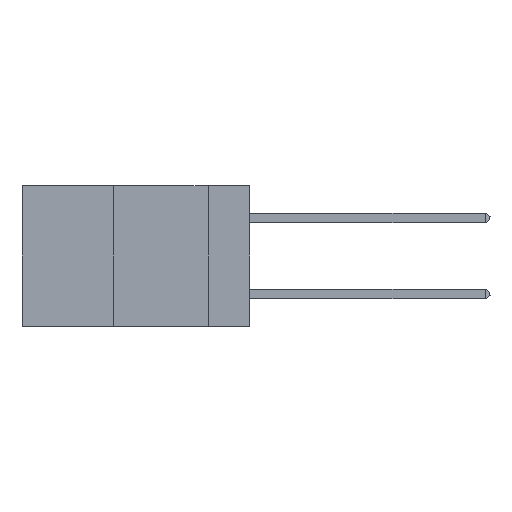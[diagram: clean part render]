
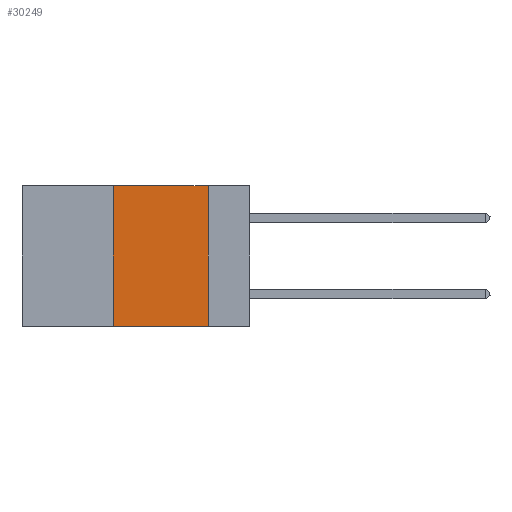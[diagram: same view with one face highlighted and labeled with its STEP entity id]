
A CAD part, left-side view. The second image highlights one B-rep face of the part: STEP entity #30249.
In plain terms, the highlighted planar face has unit normal (-1, 0, 0).
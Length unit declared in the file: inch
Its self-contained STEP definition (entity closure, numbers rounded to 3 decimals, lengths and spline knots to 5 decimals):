
#852 = VERTEX_POINT ( 'NONE', #10774 ) ;
#1862 = VERTEX_POINT ( 'NONE', #9289 ) ;
#2114 = CARTESIAN_POINT ( 'NONE',  ( 0., 0.11, -0.37 ) ) ;
#4923 = VECTOR ( 'NONE', #18340, 39.37008 ) ;
#6065 = CARTESIAN_POINT ( 'NONE',  ( 0., 0.11, 0. ) ) ;
#6107 = VERTEX_POINT ( 'NONE', #2114 ) ;
#6828 = VERTEX_POINT ( 'NONE', #16923 ) ;
#9289 = CARTESIAN_POINT ( 'NONE',  ( 0., 0.36, 0. ) ) ;
#10050 = ORIENTED_EDGE ( 'NONE', *, *, #13258, .F. ) ;
#10533 = LINE ( 'NONE', #11750, #4923 ) ;
#10774 = CARTESIAN_POINT ( 'NONE',  ( 0., 0.36, -0.37 ) ) ;
#11750 = CARTESIAN_POINT ( 'NONE',  ( 0., 0.6, 0. ) ) ;
#12560 = CARTESIAN_POINT ( 'NONE',  ( 0., 0.6, -0.37 ) ) ;
#13113 = CARTESIAN_POINT ( 'NONE',  ( 0., 0.6, 0. ) ) ;
#13258 = EDGE_CURVE ( 'NONE', #1862, #6828, #10533, .T. ) ;
#14888 = EDGE_CURVE ( 'NONE', #852, #6107, #37290, .T. ) ;
#16923 = CARTESIAN_POINT ( 'NONE',  ( 0., 0.11, 0. ) ) ;
#18340 = DIRECTION ( 'NONE',  ( 0., -1., 0. ) ) ;
#20455 = DIRECTION ( 'NONE',  ( 0., 0., -1. ) ) ;
#30249 = ADVANCED_FACE ( 'NONE', ( #44187 ), #33820, .F. ) ;
#30390 = EDGE_CURVE ( 'NONE', #6828, #6107, #40866, .T. ) ;
#31391 = EDGE_LOOP ( 'NONE', ( #43860, #10050, #34567, #35204 ) ) ;
#31463 = LINE ( 'NONE', #33371, #44222 ) ;
#33230 = DIRECTION ( 'NONE',  ( 0., 0., 1. ) ) ;
#33371 = CARTESIAN_POINT ( 'NONE',  ( 0., 0.36, 0. ) ) ;
#33820 = PLANE ( 'NONE',  #43016 ) ;
#34126 = DIRECTION ( 'NONE',  ( 1., 0., 0. ) ) ;
#34196 = VECTOR ( 'NONE', #20455, 39.37008 ) ;
#34567 = ORIENTED_EDGE ( 'NONE', *, *, #35766, .F. ) ;
#35049 = VECTOR ( 'NONE', #37935, 39.37008 ) ;
#35204 = ORIENTED_EDGE ( 'NONE', *, *, #14888, .T. ) ;
#35766 = EDGE_CURVE ( 'NONE', #852, #1862, #31463, .T. ) ;
#37290 = LINE ( 'NONE', #12560, #35049 ) ;
#37935 = DIRECTION ( 'NONE',  ( 0., -1., 0. ) ) ;
#40866 = LINE ( 'NONE', #6065, #34196 ) ;
#43016 = AXIS2_PLACEMENT_3D ( 'NONE', #13113, #34126, #44707 ) ;
#43860 = ORIENTED_EDGE ( 'NONE', *, *, #30390, .F. ) ;
#44187 = FACE_OUTER_BOUND ( 'NONE', #31391, .T. ) ;
#44222 = VECTOR ( 'NONE', #33230, 39.37008 ) ;
#44707 = DIRECTION ( 'NONE',  ( 0., 0., -1. ) ) ;
